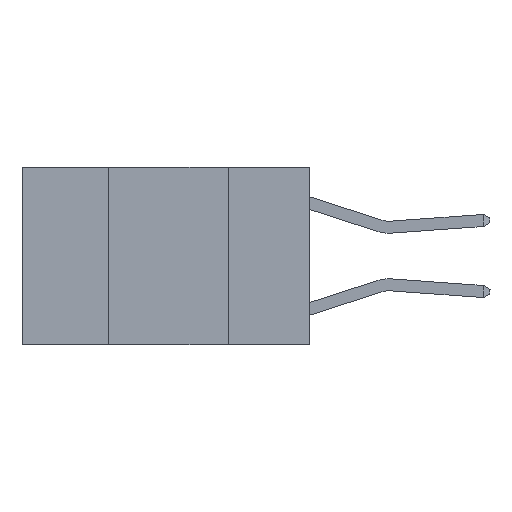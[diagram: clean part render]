
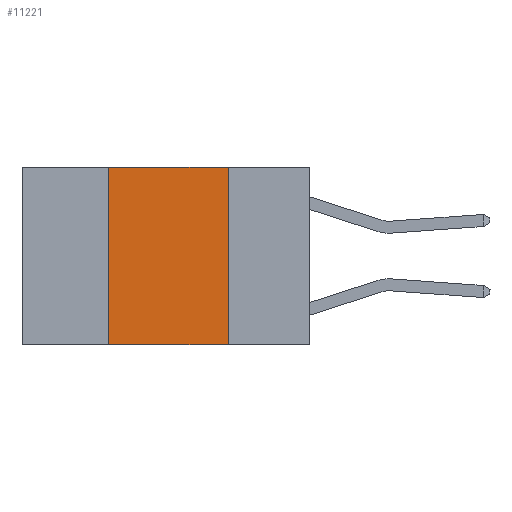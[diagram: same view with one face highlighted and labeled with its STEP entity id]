
A CAD part, left-side view. The second image highlights one B-rep face of the part: STEP entity #11221.
In plain terms, the highlighted planar face has unit normal (-1, 0, 0).
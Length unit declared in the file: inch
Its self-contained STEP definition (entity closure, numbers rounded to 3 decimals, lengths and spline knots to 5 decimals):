
#772 = DIRECTION ( 'NONE',  ( 0., 0., 1. ) ) ;
#1124 = VECTOR ( 'NONE', #11268, 39.37008 ) ;
#1269 = FACE_OUTER_BOUND ( 'NONE', #10955, .T. ) ;
#1286 = AXIS2_PLACEMENT_3D ( 'NONE', #10122, #17343, #14654 ) ;
#1501 = DIRECTION ( 'NONE',  ( 0., 0., -1. ) ) ;
#1857 = ORIENTED_EDGE ( 'NONE', *, *, #8929, .F. ) ;
#2504 = CARTESIAN_POINT ( 'NONE',  ( 0., 0.42, 0. ) ) ;
#3636 = CARTESIAN_POINT ( 'NONE',  ( 0., 0.42, 0. ) ) ;
#4676 = VERTEX_POINT ( 'NONE', #10416 ) ;
#5407 = VERTEX_POINT ( 'NONE', #3636 ) ;
#5426 = VERTEX_POINT ( 'NONE', #9785 ) ;
#6335 = EDGE_CURVE ( 'NONE', #4676, #5407, #15686, .T. ) ;
#6833 = VECTOR ( 'NONE', #772, 39.37008 ) ;
#6834 = DIRECTION ( 'NONE',  ( 0., -1., 0. ) ) ;
#7023 = LINE ( 'NONE', #17216, #8877 ) ;
#8524 = VECTOR ( 'NONE', #1501, 39.37008 ) ;
#8877 = VECTOR ( 'NONE', #6834, 39.37008 ) ;
#8929 = EDGE_CURVE ( 'NONE', #17620, #5426, #11239, .T. ) ;
#9009 = CARTESIAN_POINT ( 'NONE',  ( 0., 0.17, 0. ) ) ;
#9458 = ORIENTED_EDGE ( 'NONE', *, *, #9642, .F. ) ;
#9642 = EDGE_CURVE ( 'NONE', #5407, #17620, #16956, .T. ) ;
#9785 = CARTESIAN_POINT ( 'NONE',  ( 0., 0.17, -0.37 ) ) ;
#10122 = CARTESIAN_POINT ( 'NONE',  ( 0., 0.6, 0. ) ) ;
#10219 = PLANE ( 'NONE',  #1286 ) ;
#10416 = CARTESIAN_POINT ( 'NONE',  ( 0., 0.42, -0.37 ) ) ;
#10955 = EDGE_LOOP ( 'NONE', ( #1857, #9458, #17499, #12635 ) ) ;
#11221 = ADVANCED_FACE ( 'NONE', ( #1269 ), #10219, .F. ) ;
#11239 = LINE ( 'NONE', #9009, #8524 ) ;
#11268 = DIRECTION ( 'NONE',  ( 0., -1., 0. ) ) ;
#12525 = CARTESIAN_POINT ( 'NONE',  ( 0., 0.6, 0. ) ) ;
#12635 = ORIENTED_EDGE ( 'NONE', *, *, #15304, .T. ) ;
#13710 = CARTESIAN_POINT ( 'NONE',  ( 0., 0.17, 0. ) ) ;
#14654 = DIRECTION ( 'NONE',  ( 0., 0., -1. ) ) ;
#15304 = EDGE_CURVE ( 'NONE', #4676, #5426, #7023, .T. ) ;
#15686 = LINE ( 'NONE', #2504, #6833 ) ;
#16956 = LINE ( 'NONE', #12525, #1124 ) ;
#17216 = CARTESIAN_POINT ( 'NONE',  ( 0., 0.6, -0.37 ) ) ;
#17343 = DIRECTION ( 'NONE',  ( 1., 0., 0. ) ) ;
#17499 = ORIENTED_EDGE ( 'NONE', *, *, #6335, .F. ) ;
#17620 = VERTEX_POINT ( 'NONE', #13710 ) ;
